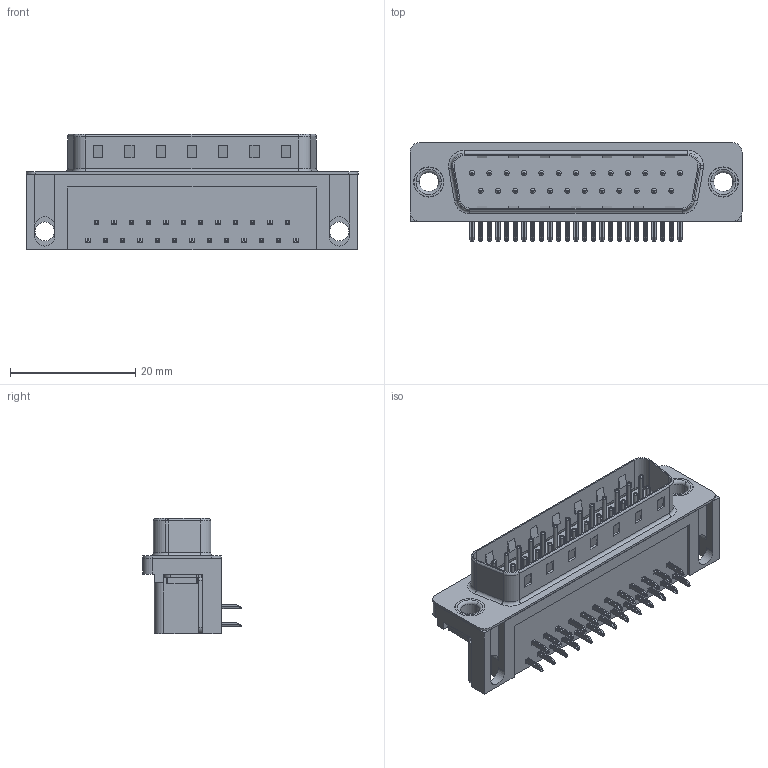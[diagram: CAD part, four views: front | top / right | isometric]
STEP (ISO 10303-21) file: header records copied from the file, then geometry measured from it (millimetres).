
FILE_DESCRIPTION (( 'STEP AP203' ), '1' );
FILE_NAME ('621-025-660-011.STEP', '2019-11-19T05:35:57', ( '' ), ( '' ), 'SwSTEP 2.0', 'SolidWorks 2016', '' );
FILE_SCHEMA (( 'CONFIG_CONTROL_DESIGN' ));
Length unit declared in the file: millimetre
Products named in the file (7): 621 Shell_25 Socket; 621 Contact Top; 621 Thru Hole Board Mount; 621 Housing_25 Socket; 621 Contact Bottom; 621 Thru Hole Rivet; 621-025-660-011
Assembly tree (31 placements, depth 2):
  621-025-660-011
    621 Housing_25 Socket
    621 Shell_25 Socket
    621 Contact Bottom  x12
    621 Contact Top  x13
    621 Thru Hole Board Mount  x2
    621 Thru Hole Rivet  x2
Bounding box: 53.04 x 15.73 x 18.4 mm (x, y, z)
Volume: 6333.4 mm3; surface area: 7646.2 mm2
Topology: 31 solids, 31 shells, 2221 faces, 5491 edges, 3389 vertices
Faces by surface type: plane 1403, cylinder 641, torus 177
Entity records: 20281 total; most frequent: DIRECTION 3322, CARTESIAN_POINT 3274, ORIENTED_EDGE 3146, EDGE_CURVE 1573, VECTOR 1136, LINE 1136, AXIS2_PLACEMENT_3D 1093, VERTEX_POINT 1009
